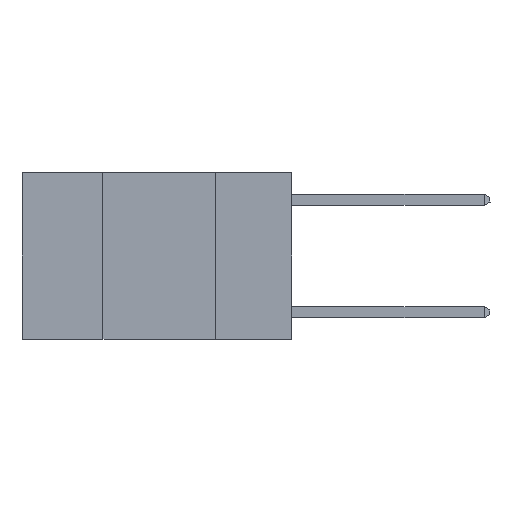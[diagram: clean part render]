
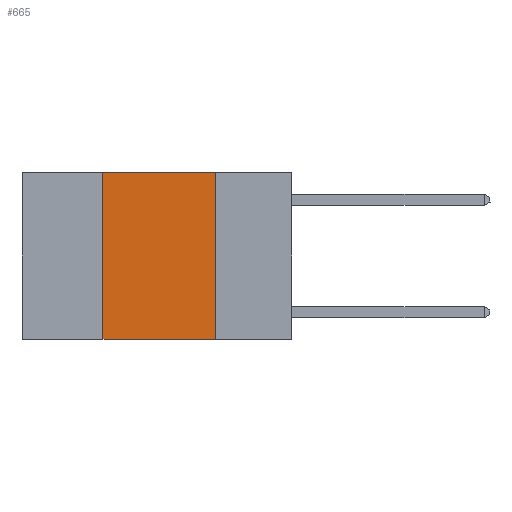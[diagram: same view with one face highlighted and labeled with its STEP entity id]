
A CAD part, left-side view. The second image highlights one B-rep face of the part: STEP entity #665.
In plain terms, the highlighted planar face has unit normal (-1, 0, 0).
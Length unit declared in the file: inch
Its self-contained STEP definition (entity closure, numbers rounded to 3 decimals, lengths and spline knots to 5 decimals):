
#110 = VERTEX_POINT ( 'NONE', #577 ) ;
#275 = CARTESIAN_POINT ( 'NONE',  ( 0., 0.42, -0.37 ) ) ;
#577 = CARTESIAN_POINT ( 'NONE',  ( 0., 0.17, 0. ) ) ;
#612 = LINE ( 'NONE', #4404, #7110 ) ;
#665 = ADVANCED_FACE ( 'NONE', ( #7278 ), #7693, .F. ) ;
#786 = DIRECTION ( 'NONE',  ( 0., 0., -1. ) ) ;
#840 = DIRECTION ( 'NONE',  ( 0., -1., 0. ) ) ;
#2023 = CARTESIAN_POINT ( 'NONE',  ( 0., 0.42, 0. ) ) ;
#2133 = VECTOR ( 'NONE', #4643, 39.37008 ) ;
#2405 = LINE ( 'NONE', #9951, #2133 ) ;
#3324 = EDGE_CURVE ( 'NONE', #5985, #110, #612, .T. ) ;
#3585 = CARTESIAN_POINT ( 'NONE',  ( 0., 0.17, -0.37 ) ) ;
#3914 = EDGE_CURVE ( 'NONE', #110, #7350, #9637, .T. ) ;
#4277 = CARTESIAN_POINT ( 'NONE',  ( 0., 0.17, 0. ) ) ;
#4404 = CARTESIAN_POINT ( 'NONE',  ( 0., 0.6, 0. ) ) ;
#4643 = DIRECTION ( 'NONE',  ( 0., 0., 1. ) ) ;
#4784 = ORIENTED_EDGE ( 'NONE', *, *, #6803, .F. ) ;
#5621 = VECTOR ( 'NONE', #786, 39.37008 ) ;
#5751 = ORIENTED_EDGE ( 'NONE', *, *, #5768, .T. ) ;
#5768 = EDGE_CURVE ( 'NONE', #7853, #7350, #10154, .T. ) ;
#5801 = ORIENTED_EDGE ( 'NONE', *, *, #3914, .F. ) ;
#5985 = VERTEX_POINT ( 'NONE', #2023 ) ;
#6691 = AXIS2_PLACEMENT_3D ( 'NONE', #9862, #6998, #7009 ) ;
#6803 = EDGE_CURVE ( 'NONE', #7853, #5985, #2405, .T. ) ;
#6998 = DIRECTION ( 'NONE',  ( 1., 0., 0. ) ) ;
#7009 = DIRECTION ( 'NONE',  ( 0., 0., -1. ) ) ;
#7110 = VECTOR ( 'NONE', #9781, 39.37008 ) ;
#7278 = FACE_OUTER_BOUND ( 'NONE', #9104, .T. ) ;
#7350 = VERTEX_POINT ( 'NONE', #3585 ) ;
#7693 = PLANE ( 'NONE',  #6691 ) ;
#7746 = VECTOR ( 'NONE', #840, 39.37008 ) ;
#7751 = ORIENTED_EDGE ( 'NONE', *, *, #3324, .F. ) ;
#7853 = VERTEX_POINT ( 'NONE', #275 ) ;
#8245 = CARTESIAN_POINT ( 'NONE',  ( 0., 0.6, -0.37 ) ) ;
#9104 = EDGE_LOOP ( 'NONE', ( #5801, #7751, #4784, #5751 ) ) ;
#9637 = LINE ( 'NONE', #4277, #5621 ) ;
#9781 = DIRECTION ( 'NONE',  ( 0., -1., 0. ) ) ;
#9862 = CARTESIAN_POINT ( 'NONE',  ( 0., 0.6, 0. ) ) ;
#9951 = CARTESIAN_POINT ( 'NONE',  ( 0., 0.42, 0. ) ) ;
#10154 = LINE ( 'NONE', #8245, #7746 ) ;
